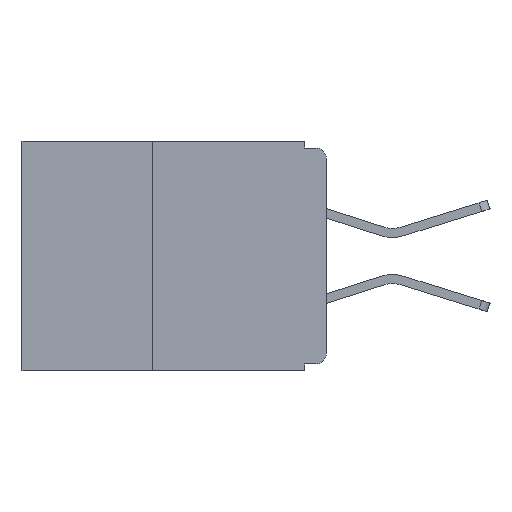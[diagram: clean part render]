
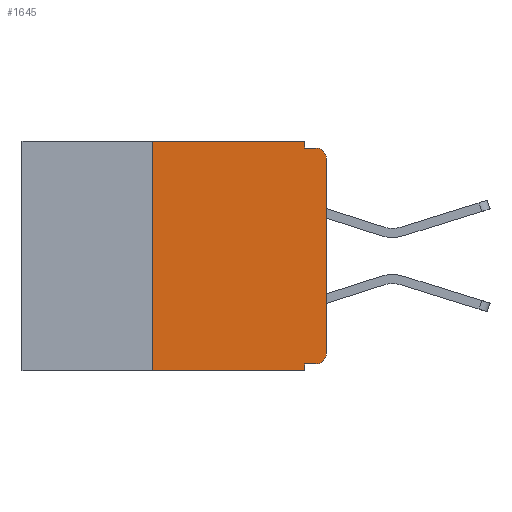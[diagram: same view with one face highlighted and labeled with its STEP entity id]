
A CAD part, left-side view. The second image highlights one B-rep face of the part: STEP entity #1645.
In plain terms, the highlighted planar face has unit normal (-1, 0, 0).
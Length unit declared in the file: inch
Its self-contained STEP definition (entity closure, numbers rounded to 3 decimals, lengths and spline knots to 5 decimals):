
#78 = LINE ( 'NONE', #4207, #12511 ) ;
#106 = ORIENTED_EDGE ( 'NONE', *, *, #3582, .F. ) ;
#199 = CARTESIAN_POINT ( 'NONE',  ( 0., 0.031, -0.33 ) ) ;
#542 = CARTESIAN_POINT ( 'NONE',  ( 0., 0.031, 0. ) ) ;
#618 = LINE ( 'NONE', #2474, #13024 ) ;
#727 = ORIENTED_EDGE ( 'NONE', *, *, #10829, .F. ) ;
#953 = VERTEX_POINT ( 'NONE', #6450 ) ;
#1447 = AXIS2_PLACEMENT_3D ( 'NONE', #3613, #15413, #6701 ) ;
#1645 = ADVANCED_FACE ( 'NONE', ( #5062 ), #15549, .F. ) ;
#1685 = EDGE_LOOP ( 'NONE', ( #10990, #11713, #3595, #3580, #3018, #727, #8088, #106, #11044, #14320 ) ) ;
#1710 = CARTESIAN_POINT ( 'NONE',  ( 0., 0., -0.025 ) ) ;
#2056 = VECTOR ( 'NONE', #10107, 39.37008 ) ;
#2057 = EDGE_CURVE ( 'NONE', #12245, #5851, #12142, .T. ) ;
#2245 = CARTESIAN_POINT ( 'NONE',  ( 0., 0.25, 0. ) ) ;
#2266 = VERTEX_POINT ( 'NONE', #1710 ) ;
#2372 = DIRECTION ( 'NONE',  ( 0., 0., -1. ) ) ;
#2474 = CARTESIAN_POINT ( 'NONE',  ( 0., 0.031, -0.33 ) ) ;
#2562 = CARTESIAN_POINT ( 'NONE',  ( 0., 0.031, -0.01 ) ) ;
#2680 = VERTEX_POINT ( 'NONE', #199 ) ;
#2827 = VERTEX_POINT ( 'NONE', #13746 ) ;
#3018 = ORIENTED_EDGE ( 'NONE', *, *, #2057, .F. ) ;
#3101 = EDGE_CURVE ( 'NONE', #12404, #953, #5017, .T. ) ;
#3288 = DIRECTION ( 'NONE',  ( -1., 0., 0. ) ) ;
#3461 = VECTOR ( 'NONE', #8616, 39.37008 ) ;
#3580 = ORIENTED_EDGE ( 'NONE', *, *, #12416, .F. ) ;
#3582 = EDGE_CURVE ( 'NONE', #12356, #2680, #618, .T. ) ;
#3595 = ORIENTED_EDGE ( 'NONE', *, *, #8472, .F. ) ;
#3613 = CARTESIAN_POINT ( 'NONE',  ( 0., 0.437, 0. ) ) ;
#3692 = CARTESIAN_POINT ( 'NONE',  ( 0., 0.031, -0.32 ) ) ;
#3988 = AXIS2_PLACEMENT_3D ( 'NONE', #9206, #9189, #9151 ) ;
#4022 = CARTESIAN_POINT ( 'NONE',  ( 0., 0.015, -0.01 ) ) ;
#4207 = CARTESIAN_POINT ( 'NONE',  ( 0., 0.25, -0.33 ) ) ;
#5017 = CIRCLE ( 'NONE', #3988, 0.015 ) ;
#5022 = CARTESIAN_POINT ( 'NONE',  ( 0., 0.031, 0. ) ) ;
#5062 = FACE_OUTER_BOUND ( 'NONE', #1685, .T. ) ;
#5320 = VECTOR ( 'NONE', #7857, 39.37008 ) ;
#5434 = DIRECTION ( 'NONE',  ( 0., 0., 1. ) ) ;
#5851 = VERTEX_POINT ( 'NONE', #542 ) ;
#5928 = VECTOR ( 'NONE', #7125, 39.37008 ) ;
#6009 = EDGE_CURVE ( 'NONE', #2827, #2680, #6325, .T. ) ;
#6233 = CARTESIAN_POINT ( 'NONE',  ( 0., 0.015, -0.32 ) ) ;
#6313 = VERTEX_POINT ( 'NONE', #4022 ) ;
#6325 = LINE ( 'NONE', #13034, #5928 ) ;
#6450 = CARTESIAN_POINT ( 'NONE',  ( 0., 0., -0.305 ) ) ;
#6567 = EDGE_CURVE ( 'NONE', #953, #2266, #7641, .T. ) ;
#6681 = DIRECTION ( 'NONE',  ( 0., -1., 0. ) ) ;
#6686 = LINE ( 'NONE', #5022, #3461 ) ;
#6701 = DIRECTION ( 'NONE',  ( 0., 0., -1. ) ) ;
#7125 = DIRECTION ( 'NONE',  ( 0., -1., 0. ) ) ;
#7641 = LINE ( 'NONE', #12867, #13569 ) ;
#7857 = DIRECTION ( 'NONE',  ( 0., 1., 0. ) ) ;
#7974 = EDGE_CURVE ( 'NONE', #2266, #6313, #15181, .T. ) ;
#8088 = ORIENTED_EDGE ( 'NONE', *, *, #6009, .T. ) ;
#8472 = EDGE_CURVE ( 'NONE', #13032, #6313, #11645, .T. ) ;
#8616 = DIRECTION ( 'NONE',  ( 0., 0., -1. ) ) ;
#8918 = CARTESIAN_POINT ( 'NONE',  ( 0., 0., -0.01 ) ) ;
#9151 = DIRECTION ( 'NONE',  ( 0., 0., -1. ) ) ;
#9189 = DIRECTION ( 'NONE',  ( -1., 0., 0. ) ) ;
#9206 = CARTESIAN_POINT ( 'NONE',  ( 0., 0.015, -0.305 ) ) ;
#9378 = VECTOR ( 'NONE', #6681, 39.37008 ) ;
#10107 = DIRECTION ( 'NONE',  ( 0., -1., 0. ) ) ;
#10486 = CARTESIAN_POINT ( 'NONE',  ( 0., 0.015, -0.025 ) ) ;
#10829 = EDGE_CURVE ( 'NONE', #2827, #12245, #78, .T. ) ;
#10990 = ORIENTED_EDGE ( 'NONE', *, *, #6567, .T. ) ;
#11044 = ORIENTED_EDGE ( 'NONE', *, *, #13531, .F. ) ;
#11285 = AXIS2_PLACEMENT_3D ( 'NONE', #10486, #3288, #11664 ) ;
#11645 = LINE ( 'NONE', #8918, #2056 ) ;
#11664 = DIRECTION ( 'NONE',  ( 0., 0., -1. ) ) ;
#11666 = DIRECTION ( 'NONE',  ( 0., 0., 1. ) ) ;
#11713 = ORIENTED_EDGE ( 'NONE', *, *, #7974, .T. ) ;
#12142 = LINE ( 'NONE', #14992, #9378 ) ;
#12245 = VERTEX_POINT ( 'NONE', #2245 ) ;
#12356 = VERTEX_POINT ( 'NONE', #3692 ) ;
#12404 = VERTEX_POINT ( 'NONE', #6233 ) ;
#12416 = EDGE_CURVE ( 'NONE', #5851, #13032, #6686, .T. ) ;
#12511 = VECTOR ( 'NONE', #5434, 39.37008 ) ;
#12867 = CARTESIAN_POINT ( 'NONE',  ( 0., 0., 0. ) ) ;
#13024 = VECTOR ( 'NONE', #2372, 39.37008 ) ;
#13032 = VERTEX_POINT ( 'NONE', #2562 ) ;
#13034 = CARTESIAN_POINT ( 'NONE',  ( 0., 0.437, -0.33 ) ) ;
#13531 = EDGE_CURVE ( 'NONE', #12404, #12356, #14829, .T. ) ;
#13569 = VECTOR ( 'NONE', #11666, 39.37008 ) ;
#13746 = CARTESIAN_POINT ( 'NONE',  ( 0., 0.25, -0.33 ) ) ;
#14320 = ORIENTED_EDGE ( 'NONE', *, *, #3101, .T. ) ;
#14829 = LINE ( 'NONE', #14938, #5320 ) ;
#14938 = CARTESIAN_POINT ( 'NONE',  ( 0., 0., -0.32 ) ) ;
#14992 = CARTESIAN_POINT ( 'NONE',  ( 0., 0.437, 0. ) ) ;
#15181 = CIRCLE ( 'NONE', #11285, 0.015 ) ;
#15413 = DIRECTION ( 'NONE',  ( 1., 0., 0. ) ) ;
#15549 = PLANE ( 'NONE',  #1447 ) ;
